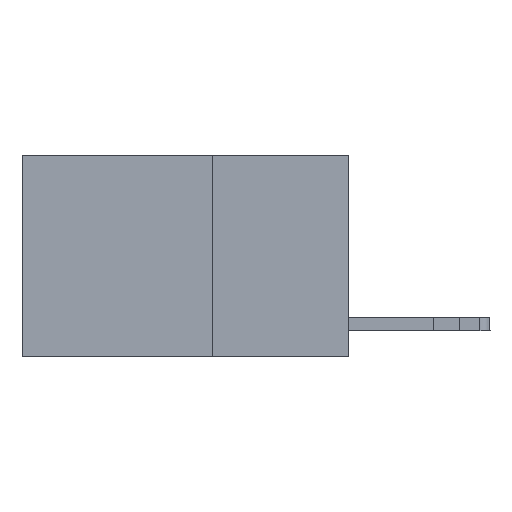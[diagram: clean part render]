
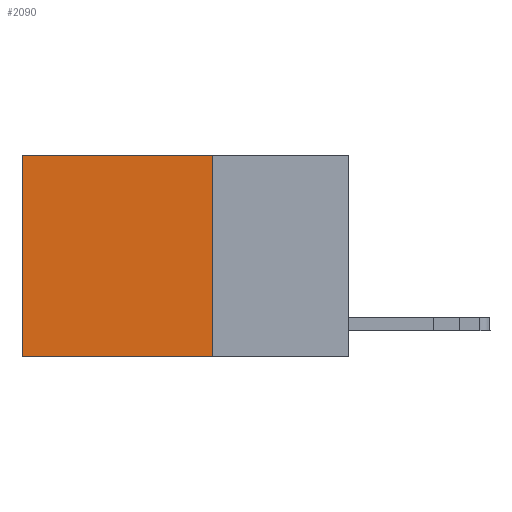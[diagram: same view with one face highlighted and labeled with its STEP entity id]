
A CAD part, left-side view. The second image highlights one B-rep face of the part: STEP entity #2090.
In plain terms, the highlighted planar face has unit normal (-1, 0, 0).
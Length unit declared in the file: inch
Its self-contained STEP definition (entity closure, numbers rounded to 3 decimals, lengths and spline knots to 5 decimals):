
#11 = DIRECTION ( 'NONE',  ( 0., 1., 0. ) ) ;
#45 = CARTESIAN_POINT ( 'NONE',  ( 0.2625, 0.6, 0. ) ) ;
#553 = AXIS2_PLACEMENT_3D ( 'NONE', #7222, #2258, #3252 ) ;
#960 = CARTESIAN_POINT ( 'NONE',  ( 0.2625, 0.25, -0.37 ) ) ;
#1102 = ORIENTED_EDGE ( 'NONE', *, *, #11381, .T. ) ;
#2090 = ADVANCED_FACE ( 'NONE', ( #6308 ), #7159, .F. ) ;
#2258 = DIRECTION ( 'NONE',  ( 1., 0., 0. ) ) ;
#3252 = DIRECTION ( 'NONE',  ( 0., 0., -1. ) ) ;
#3777 = VECTOR ( 'NONE', #4478, 39.37008 ) ;
#4286 = LINE ( 'NONE', #8266, #3777 ) ;
#4415 = DIRECTION ( 'NONE',  ( 0., 0., -1. ) ) ;
#4478 = DIRECTION ( 'NONE',  ( 0., 1., 0. ) ) ;
#4521 = ORIENTED_EDGE ( 'NONE', *, *, #10451, .F. ) ;
#5268 = ORIENTED_EDGE ( 'NONE', *, *, #5895, .F. ) ;
#5347 = CARTESIAN_POINT ( 'NONE',  ( 0.2625, 0.25, 0. ) ) ;
#5730 = VERTEX_POINT ( 'NONE', #6516 ) ;
#5895 = EDGE_CURVE ( 'NONE', #6119, #7547, #9483, .T. ) ;
#6119 = VERTEX_POINT ( 'NONE', #6283 ) ;
#6283 = CARTESIAN_POINT ( 'NONE',  ( 0.2625, 0.25, -0.37 ) ) ;
#6308 = FACE_OUTER_BOUND ( 'NONE', #12321, .T. ) ;
#6516 = CARTESIAN_POINT ( 'NONE',  ( 0.2625, 0.25, 0. ) ) ;
#7159 = PLANE ( 'NONE',  #553 ) ;
#7222 = CARTESIAN_POINT ( 'NONE',  ( 0.2625, 0.25, 0. ) ) ;
#7547 = VERTEX_POINT ( 'NONE', #11406 ) ;
#7764 = VECTOR ( 'NONE', #8603, 39.37008 ) ;
#7902 = CARTESIAN_POINT ( 'NONE',  ( 0.2625, 0.6, 0. ) ) ;
#8266 = CARTESIAN_POINT ( 'NONE',  ( 0.2625, 0.25, 0. ) ) ;
#8603 = DIRECTION ( 'NONE',  ( 0., 0., -1. ) ) ;
#8723 = ORIENTED_EDGE ( 'NONE', *, *, #10411, .T. ) ;
#8936 = VECTOR ( 'NONE', #4415, 39.37008 ) ;
#9017 = VECTOR ( 'NONE', #11, 39.37008 ) ;
#9483 = LINE ( 'NONE', #960, #9017 ) ;
#9714 = LINE ( 'NONE', #45, #7764 ) ;
#10177 = LINE ( 'NONE', #5347, #8936 ) ;
#10411 = EDGE_CURVE ( 'NONE', #5730, #11815, #4286, .T. ) ;
#10451 = EDGE_CURVE ( 'NONE', #5730, #6119, #10177, .T. ) ;
#11381 = EDGE_CURVE ( 'NONE', #11815, #7547, #9714, .T. ) ;
#11406 = CARTESIAN_POINT ( 'NONE',  ( 0.2625, 0.6, -0.37 ) ) ;
#11815 = VERTEX_POINT ( 'NONE', #7902 ) ;
#12321 = EDGE_LOOP ( 'NONE', ( #1102, #5268, #4521, #8723 ) ) ;
